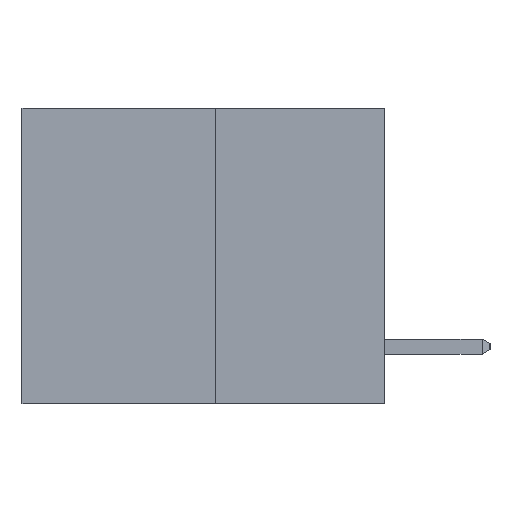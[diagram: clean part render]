
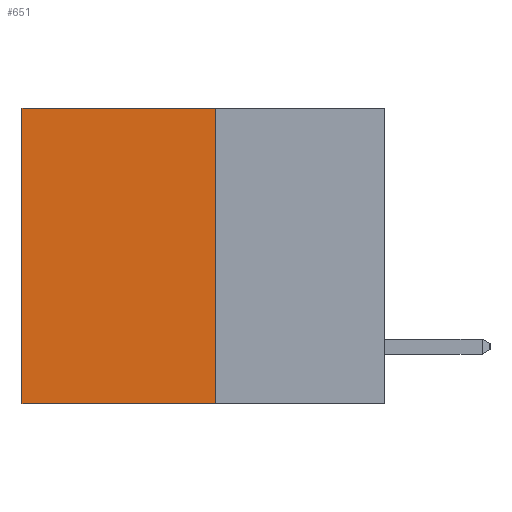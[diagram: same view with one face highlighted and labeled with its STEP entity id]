
A CAD part, left-side view. The second image highlights one B-rep face of the part: STEP entity #651.
In plain terms, the highlighted planar face has unit normal (-1, 0, 0).
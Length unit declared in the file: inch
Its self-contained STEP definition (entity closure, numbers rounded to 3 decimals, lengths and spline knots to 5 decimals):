
#359 = VERTEX_POINT ( 'NONE', #678 ) ;
#558 = DIRECTION ( 'NONE',  ( 0., 1., 0. ) ) ;
#651 = ADVANCED_FACE ( 'NONE', ( #16873 ), #6085, .F. ) ;
#678 = CARTESIAN_POINT ( 'NONE',  ( 0.3165, 0.28, 0. ) ) ;
#1064 = VERTEX_POINT ( 'NONE', #1172 ) ;
#1144 = DIRECTION ( 'NONE',  ( 0., 1., 0. ) ) ;
#1172 = CARTESIAN_POINT ( 'NONE',  ( 0.3165, 0.28, -0.49 ) ) ;
#1333 = CARTESIAN_POINT ( 'NONE',  ( 0.3165, 0.28, 0. ) ) ;
#2624 = EDGE_CURVE ( 'NONE', #1064, #15168, #14386, .T. ) ;
#3152 = DIRECTION ( 'NONE',  ( 0., 0., -1. ) ) ;
#3516 = EDGE_CURVE ( 'NONE', #8786, #15168, #19350, .T. ) ;
#3763 = CARTESIAN_POINT ( 'NONE',  ( 0.3165, 0.6, -0.49 ) ) ;
#3881 = CARTESIAN_POINT ( 'NONE',  ( 0.3165, 0.28, -0.49 ) ) ;
#4423 = VECTOR ( 'NONE', #16077, 39.37008 ) ;
#4561 = EDGE_CURVE ( 'NONE', #359, #8786, #13773, .T. ) ;
#6085 = PLANE ( 'NONE',  #11978 ) ;
#7712 = DIRECTION ( 'NONE',  ( 1., 0., 0. ) ) ;
#8283 = CARTESIAN_POINT ( 'NONE',  ( 0.3165, 0.6, -0.49 ) ) ;
#8536 = DIRECTION ( 'NONE',  ( 0., 0., -1. ) ) ;
#8786 = VERTEX_POINT ( 'NONE', #16810 ) ;
#9234 = ORIENTED_EDGE ( 'NONE', *, *, #2624, .F. ) ;
#9293 = EDGE_CURVE ( 'NONE', #359, #1064, #9957, .T. ) ;
#9957 = LINE ( 'NONE', #3881, #11915 ) ;
#10994 = VECTOR ( 'NONE', #558, 39.37008 ) ;
#11177 = ORIENTED_EDGE ( 'NONE', *, *, #4561, .T. ) ;
#11674 = ORIENTED_EDGE ( 'NONE', *, *, #9293, .F. ) ;
#11915 = VECTOR ( 'NONE', #8536, 39.37008 ) ;
#11978 = AXIS2_PLACEMENT_3D ( 'NONE', #15397, #7712, #3152 ) ;
#13159 = EDGE_LOOP ( 'NONE', ( #16591, #9234, #11674, #11177 ) ) ;
#13773 = LINE ( 'NONE', #1333, #15465 ) ;
#14386 = LINE ( 'NONE', #14433, #10994 ) ;
#14433 = CARTESIAN_POINT ( 'NONE',  ( 0.3165, 0.28, -0.49 ) ) ;
#15168 = VERTEX_POINT ( 'NONE', #8283 ) ;
#15397 = CARTESIAN_POINT ( 'NONE',  ( 0.3165, 0.28, -0.49 ) ) ;
#15465 = VECTOR ( 'NONE', #1144, 39.37008 ) ;
#16077 = DIRECTION ( 'NONE',  ( 0., 0., -1. ) ) ;
#16591 = ORIENTED_EDGE ( 'NONE', *, *, #3516, .T. ) ;
#16810 = CARTESIAN_POINT ( 'NONE',  ( 0.3165, 0.6, 0. ) ) ;
#16873 = FACE_OUTER_BOUND ( 'NONE', #13159, .T. ) ;
#19350 = LINE ( 'NONE', #3763, #4423 ) ;
